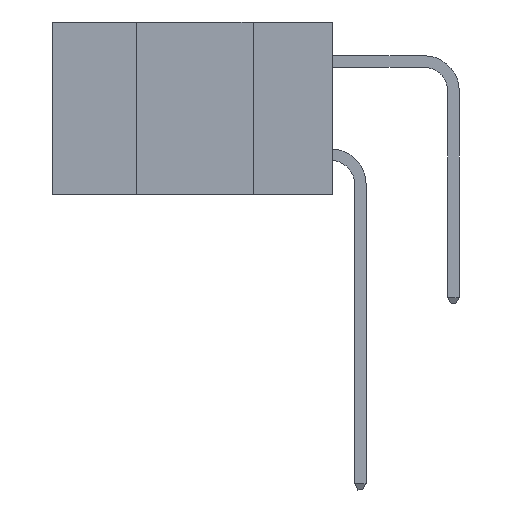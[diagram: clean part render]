
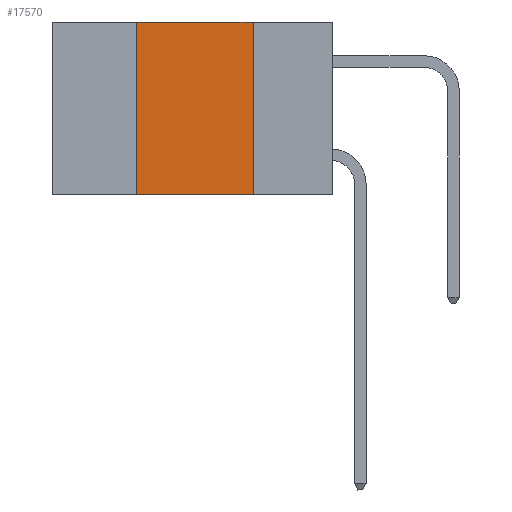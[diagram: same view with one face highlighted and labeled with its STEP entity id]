
A CAD part, left-side view. The second image highlights one B-rep face of the part: STEP entity #17570.
In plain terms, the highlighted planar face has unit normal (-1, 0, 0).
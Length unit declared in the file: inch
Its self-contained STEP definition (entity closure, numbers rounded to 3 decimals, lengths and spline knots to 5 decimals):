
#535 = CARTESIAN_POINT ( 'NONE',  ( 0., 0.17, -0.37 ) ) ;
#735 = ORIENTED_EDGE ( 'NONE', *, *, #16564, .F. ) ;
#1574 = AXIS2_PLACEMENT_3D ( 'NONE', #22064, #10453, #23970 ) ;
#2254 = VERTEX_POINT ( 'NONE', #13469 ) ;
#2661 = CARTESIAN_POINT ( 'NONE',  ( 0., 0.17, -0.37 ) ) ;
#2729 = DIRECTION ( 'NONE',  ( 0., 0., 1. ) ) ;
#2896 = VECTOR ( 'NONE', #2729, 39.37008 ) ;
#3844 = DIRECTION ( 'NONE',  ( 0., -1., 0. ) ) ;
#4375 = VERTEX_POINT ( 'NONE', #535 ) ;
#5554 = ORIENTED_EDGE ( 'NONE', *, *, #12685, .F. ) ;
#5628 = CARTESIAN_POINT ( 'NONE',  ( 0., 0.6, 0. ) ) ;
#5678 = VERTEX_POINT ( 'NONE', #16202 ) ;
#5741 = VECTOR ( 'NONE', #10730, 39.37008 ) ;
#7103 = VECTOR ( 'NONE', #3844, 39.37008 ) ;
#7669 = EDGE_LOOP ( 'NONE', ( #11686, #735, #5554, #20505 ) ) ;
#7681 = DIRECTION ( 'NONE',  ( 0., -1., 0. ) ) ;
#10453 = DIRECTION ( 'NONE',  ( 1., 0., 0. ) ) ;
#10730 = DIRECTION ( 'NONE',  ( 0., 0., -1. ) ) ;
#11352 = EDGE_CURVE ( 'NONE', #13999, #4375, #22080, .T. ) ;
#11686 = ORIENTED_EDGE ( 'NONE', *, *, #17874, .F. ) ;
#12654 = FACE_OUTER_BOUND ( 'NONE', #7669, .T. ) ;
#12685 = EDGE_CURVE ( 'NONE', #13999, #2254, #17413, .T. ) ;
#13469 = CARTESIAN_POINT ( 'NONE',  ( 0., 0.42, 0. ) ) ;
#13775 = CARTESIAN_POINT ( 'NONE',  ( 0., 0.6, -0.37 ) ) ;
#13999 = VERTEX_POINT ( 'NONE', #21226 ) ;
#14253 = VECTOR ( 'NONE', #7681, 39.37008 ) ;
#14847 = LINE ( 'NONE', #5628, #14253 ) ;
#16202 = CARTESIAN_POINT ( 'NONE',  ( 0., 0.17, 0. ) ) ;
#16222 = PLANE ( 'NONE',  #1574 ) ;
#16564 = EDGE_CURVE ( 'NONE', #2254, #5678, #14847, .T. ) ;
#17413 = LINE ( 'NONE', #23511, #2896 ) ;
#17570 = ADVANCED_FACE ( 'NONE', ( #12654 ), #16222, .F. ) ;
#17874 = EDGE_CURVE ( 'NONE', #5678, #4375, #21397, .T. ) ;
#20505 = ORIENTED_EDGE ( 'NONE', *, *, #11352, .T. ) ;
#21226 = CARTESIAN_POINT ( 'NONE',  ( 0., 0.42, -0.37 ) ) ;
#21397 = LINE ( 'NONE', #2661, #5741 ) ;
#22064 = CARTESIAN_POINT ( 'NONE',  ( 0., 0.6, 0. ) ) ;
#22080 = LINE ( 'NONE', #13775, #7103 ) ;
#23511 = CARTESIAN_POINT ( 'NONE',  ( 0., 0.42, -0.37 ) ) ;
#23970 = DIRECTION ( 'NONE',  ( 0., 0., -1. ) ) ;
